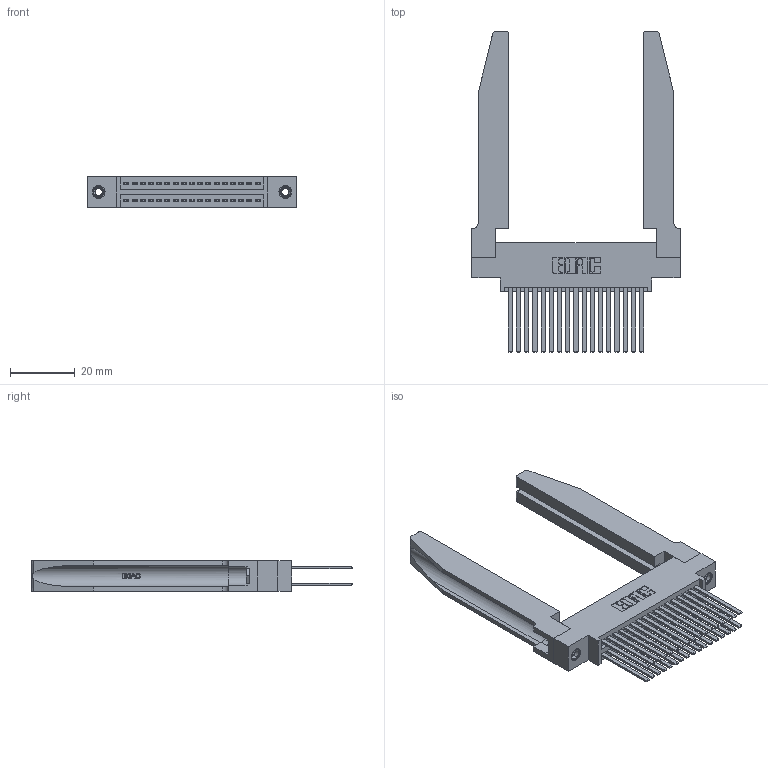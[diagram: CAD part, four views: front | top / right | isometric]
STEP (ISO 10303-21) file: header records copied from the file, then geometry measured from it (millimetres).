
FILE_DESCRIPTION (( 'STEP AP203' ), '1' );
FILE_NAME ('395-034-544-878.STEP', '2019-10-17T18:06:50', ( '' ), ( '' ), 'SwSTEP 2.0', 'SolidWorks 2016', '' );
FILE_SCHEMA (( 'CONFIG_CONTROL_DESIGN' ));
Length unit declared in the file: inch
Products named in the file (5): 345-220-078_345-220-078; 395-034-544-878; 345 Part_0.170 Offset - 0.156 Dia-TH; 345-292-001_345-293-144; 345-250-001_345-250-001-102
Assembly tree (39 placements, depth 2):
  395-034-544-878
    345 Part_0.170 Offset - 0.156 Dia-TH
    345-292-001_345-293-144  x34
    345-250-001_345-250-001-102  x2
    345-220-078_345-220-078  x2
Bounding box: 64.41 x 99.24 x 9.4 mm (x, y, z)
Volume: 14158.9 mm3; surface area: 17337.9 mm2
Topology: 39 solids, 39 shells, 1860 faces, 5415 edges, 3554 vertices
Faces by surface type: plane 1212, cylinder 596, bspline 36, cone 12, torus 4
Entity records: 21392 total; most frequent: CARTESIAN_POINT 4527, ORIENTED_EDGE 3358, DIRECTION 3013, EDGE_CURVE 1679, LINE 1389, VECTOR 1389, VERTEX_POINT 1112, AXIS2_PLACEMENT_3D 812
